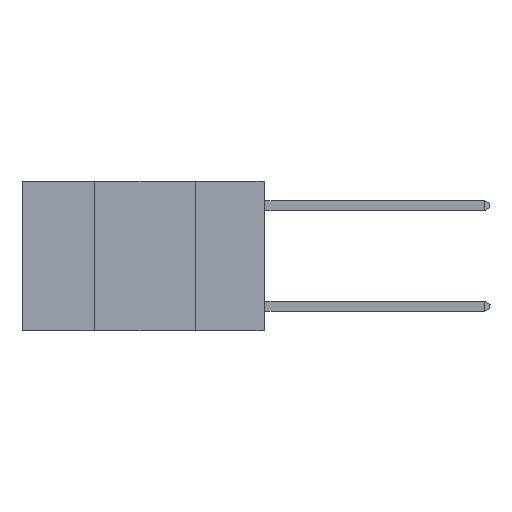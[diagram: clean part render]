
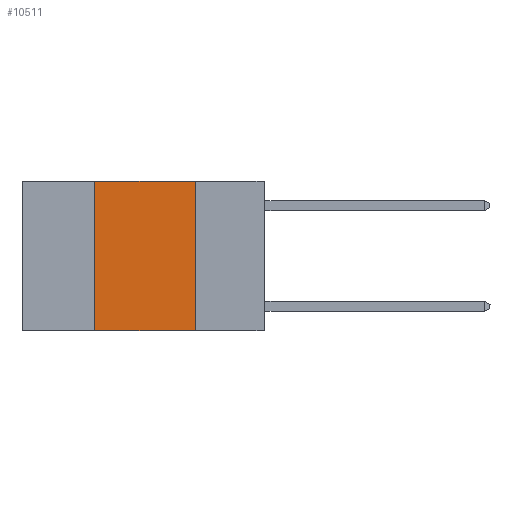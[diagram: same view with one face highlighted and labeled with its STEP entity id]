
A CAD part, left-side view. The second image highlights one B-rep face of the part: STEP entity #10511.
In plain terms, the highlighted planar face has unit normal (-1, 0, 0).
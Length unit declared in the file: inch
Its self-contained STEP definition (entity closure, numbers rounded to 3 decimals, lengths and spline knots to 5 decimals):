
#645 = DIRECTION ( 'NONE',  ( 0., 0., 1. ) ) ;
#692 = EDGE_CURVE ( 'NONE', #7115, #3663, #13550, .T. ) ;
#1598 = CARTESIAN_POINT ( 'NONE',  ( 0., 0.6, 0. ) ) ;
#1907 = EDGE_CURVE ( 'NONE', #4323, #8396, #7526, .T. ) ;
#2067 = CARTESIAN_POINT ( 'NONE',  ( 0., 0.17, 0. ) ) ;
#3643 = DIRECTION ( 'NONE',  ( 0., -1., 0. ) ) ;
#3663 = VERTEX_POINT ( 'NONE', #2067 ) ;
#3787 = LINE ( 'NONE', #11670, #9641 ) ;
#4248 = CARTESIAN_POINT ( 'NONE',  ( 0., 0.42, -0.37 ) ) ;
#4323 = VERTEX_POINT ( 'NONE', #4248 ) ;
#4815 = VECTOR ( 'NONE', #7096, 39.37008 ) ;
#6222 = PLANE ( 'NONE',  #6528 ) ;
#6269 = DIRECTION ( 'NONE',  ( 0., 0., -1. ) ) ;
#6528 = AXIS2_PLACEMENT_3D ( 'NONE', #10654, #12831, #6269 ) ;
#6806 = ORIENTED_EDGE ( 'NONE', *, *, #692, .F. ) ;
#7096 = DIRECTION ( 'NONE',  ( 0., -1., 0. ) ) ;
#7115 = VERTEX_POINT ( 'NONE', #9179 ) ;
#7187 = VECTOR ( 'NONE', #3643, 39.37008 ) ;
#7465 = LINE ( 'NONE', #13324, #10065 ) ;
#7526 = LINE ( 'NONE', #8079, #7187 ) ;
#7880 = DIRECTION ( 'NONE',  ( 0., 0., -1. ) ) ;
#8079 = CARTESIAN_POINT ( 'NONE',  ( 0., 0.6, -0.37 ) ) ;
#8396 = VERTEX_POINT ( 'NONE', #10316 ) ;
#9179 = CARTESIAN_POINT ( 'NONE',  ( 0., 0.42, 0. ) ) ;
#9641 = VECTOR ( 'NONE', #645, 39.37008 ) ;
#9725 = ORIENTED_EDGE ( 'NONE', *, *, #14118, .F. ) ;
#10065 = VECTOR ( 'NONE', #7880, 39.37008 ) ;
#10077 = ORIENTED_EDGE ( 'NONE', *, *, #1907, .T. ) ;
#10316 = CARTESIAN_POINT ( 'NONE',  ( 0., 0.17, -0.37 ) ) ;
#10511 = ADVANCED_FACE ( 'NONE', ( #13474 ), #6222, .F. ) ;
#10654 = CARTESIAN_POINT ( 'NONE',  ( 0., 0.6, 0. ) ) ;
#10693 = EDGE_LOOP ( 'NONE', ( #12308, #6806, #9725, #10077 ) ) ;
#11670 = CARTESIAN_POINT ( 'NONE',  ( 0., 0.42, 0. ) ) ;
#11962 = EDGE_CURVE ( 'NONE', #3663, #8396, #7465, .T. ) ;
#12308 = ORIENTED_EDGE ( 'NONE', *, *, #11962, .F. ) ;
#12831 = DIRECTION ( 'NONE',  ( 1., 0., 0. ) ) ;
#13324 = CARTESIAN_POINT ( 'NONE',  ( 0., 0.17, 0. ) ) ;
#13474 = FACE_OUTER_BOUND ( 'NONE', #10693, .T. ) ;
#13550 = LINE ( 'NONE', #1598, #4815 ) ;
#14118 = EDGE_CURVE ( 'NONE', #4323, #7115, #3787, .T. ) ;
